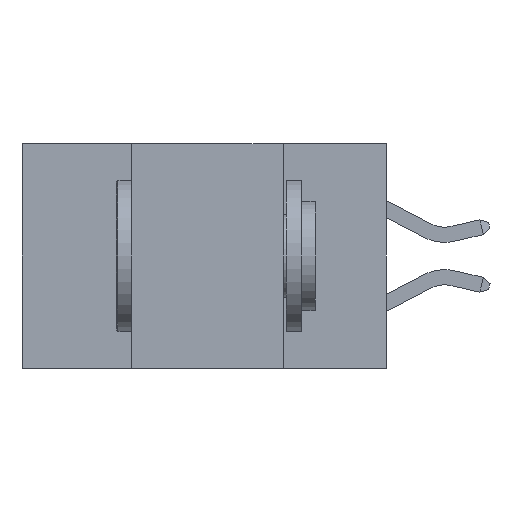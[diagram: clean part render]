
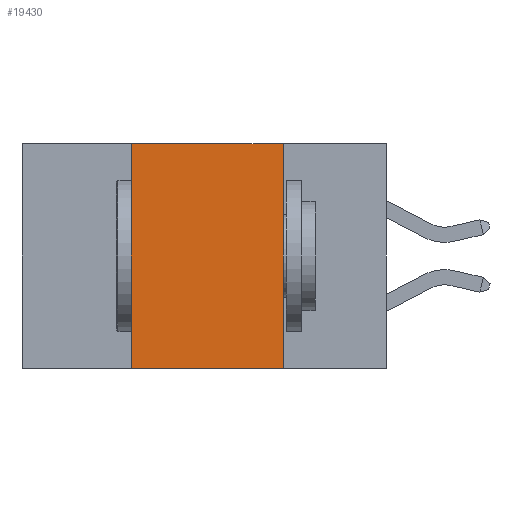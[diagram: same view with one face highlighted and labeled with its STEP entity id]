
A CAD part, left-side view. The second image highlights one B-rep face of the part: STEP entity #19430.
In plain terms, the highlighted planar face has unit normal (-1, 0, 0).
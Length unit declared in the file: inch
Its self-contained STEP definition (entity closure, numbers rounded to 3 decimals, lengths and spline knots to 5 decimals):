
#157 = VECTOR ( 'NONE', #22538, 39.37008 ) ;
#1055 = DIRECTION ( 'NONE',  ( 1., 0., 0. ) ) ;
#1359 = EDGE_CURVE ( 'NONE', #22169, #21112, #21957, .T. ) ;
#2136 = FACE_OUTER_BOUND ( 'NONE', #24065, .T. ) ;
#2411 = VECTOR ( 'NONE', #23410, 39.37008 ) ;
#2452 = DIRECTION ( 'NONE',  ( 0., 0., 1. ) ) ;
#3175 = CARTESIAN_POINT ( 'NONE',  ( 0., 0.6, 0. ) ) ;
#4507 = EDGE_CURVE ( 'NONE', #21112, #22870, #13594, .T. ) ;
#5012 = CARTESIAN_POINT ( 'NONE',  ( 0., 0.6, -0.37 ) ) ;
#5492 = EDGE_CURVE ( 'NONE', #13015, #22169, #11759, .T. ) ;
#6135 = VECTOR ( 'NONE', #16283, 39.37008 ) ;
#6211 = EDGE_CURVE ( 'NONE', #13015, #22870, #23318, .T. ) ;
#6588 = VECTOR ( 'NONE', #2452, 39.37008 ) ;
#7020 = AXIS2_PLACEMENT_3D ( 'NONE', #3175, #1055, #14629 ) ;
#8458 = CARTESIAN_POINT ( 'NONE',  ( 0., 0.42, 0. ) ) ;
#8738 = ORIENTED_EDGE ( 'NONE', *, *, #6211, .T. ) ;
#8762 = ORIENTED_EDGE ( 'NONE', *, *, #5492, .F. ) ;
#9790 = CARTESIAN_POINT ( 'NONE',  ( 0., 0.17, 0. ) ) ;
#10309 = CARTESIAN_POINT ( 'NONE',  ( 0., 0.42, 0. ) ) ;
#11759 = LINE ( 'NONE', #8458, #6588 ) ;
#13015 = VERTEX_POINT ( 'NONE', #20187 ) ;
#13594 = LINE ( 'NONE', #9790, #2411 ) ;
#14629 = DIRECTION ( 'NONE',  ( 0., 0., -1. ) ) ;
#15008 = CARTESIAN_POINT ( 'NONE',  ( 0., 0.17, -0.37 ) ) ;
#16283 = DIRECTION ( 'NONE',  ( 0., -1., 0. ) ) ;
#19430 = ADVANCED_FACE ( 'NONE', ( #2136 ), #24490, .F. ) ;
#20187 = CARTESIAN_POINT ( 'NONE',  ( 0., 0.42, -0.37 ) ) ;
#21112 = VERTEX_POINT ( 'NONE', #21850 ) ;
#21850 = CARTESIAN_POINT ( 'NONE',  ( 0., 0.17, 0. ) ) ;
#21957 = LINE ( 'NONE', #24385, #6135 ) ;
#22169 = VERTEX_POINT ( 'NONE', #10309 ) ;
#22538 = DIRECTION ( 'NONE',  ( 0., -1., 0. ) ) ;
#22870 = VERTEX_POINT ( 'NONE', #15008 ) ;
#23311 = ORIENTED_EDGE ( 'NONE', *, *, #1359, .F. ) ;
#23318 = LINE ( 'NONE', #5012, #157 ) ;
#23410 = DIRECTION ( 'NONE',  ( 0., 0., -1. ) ) ;
#24065 = EDGE_LOOP ( 'NONE', ( #24370, #23311, #8762, #8738 ) ) ;
#24370 = ORIENTED_EDGE ( 'NONE', *, *, #4507, .F. ) ;
#24385 = CARTESIAN_POINT ( 'NONE',  ( 0., 0.6, 0. ) ) ;
#24490 = PLANE ( 'NONE',  #7020 ) ;
